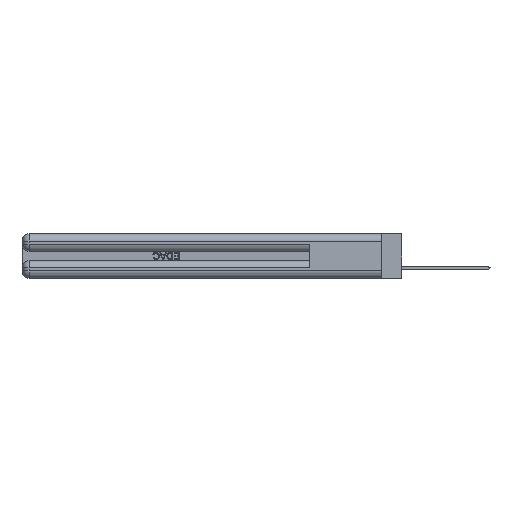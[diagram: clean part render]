
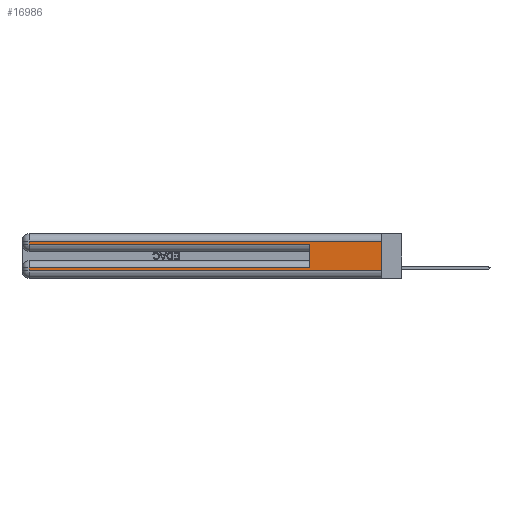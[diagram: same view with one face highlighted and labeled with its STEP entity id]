
A CAD part, left-side view. The second image highlights one B-rep face of the part: STEP entity #16986.
In plain terms, the highlighted planar face has unit normal (-1, 0, 0).
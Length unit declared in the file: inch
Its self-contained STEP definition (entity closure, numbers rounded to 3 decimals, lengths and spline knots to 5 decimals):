
#219 = EDGE_CURVE ( 'NONE', #20046, #39819, #32387, .T. ) ;
#1329 = ORIENTED_EDGE ( 'NONE', *, *, #219, .F. ) ;
#1887 = CARTESIAN_POINT ( 'NONE',  ( 0., 2.94, 0.37 ) ) ;
#1982 = AXIS2_PLACEMENT_3D ( 'NONE', #4326, #38796, #10562 ) ;
#2316 = CARTESIAN_POINT ( 'NONE',  ( 0., 0., 0.285 ) ) ;
#2643 = VECTOR ( 'NONE', #18544, 39.37008 ) ;
#3622 = DIRECTION ( 'NONE',  ( 0., 0., -1. ) ) ;
#4110 = VERTEX_POINT ( 'NONE', #21981 ) ;
#4326 = CARTESIAN_POINT ( 'NONE',  ( 0., 0., 0.37 ) ) ;
#4885 = VECTOR ( 'NONE', #17716, 39.37008 ) ;
#5286 = LINE ( 'NONE', #22515, #23518 ) ;
#6359 = ORIENTED_EDGE ( 'NONE', *, *, #16878, .T. ) ;
#6873 = VERTEX_POINT ( 'NONE', #15653 ) ;
#8966 = VERTEX_POINT ( 'NONE', #26097 ) ;
#9294 = ORIENTED_EDGE ( 'NONE', *, *, #29527, .T. ) ;
#9932 = EDGE_CURVE ( 'NONE', #8966, #39819, #20279, .T. ) ;
#10562 = DIRECTION ( 'NONE',  ( 0., 0., -1. ) ) ;
#11868 = VERTEX_POINT ( 'NONE', #23362 ) ;
#11932 = VECTOR ( 'NONE', #17241, 39.37008 ) ;
#13137 = ORIENTED_EDGE ( 'NONE', *, *, #9932, .T. ) ;
#13604 = DIRECTION ( 'NONE',  ( 0., 0., -1. ) ) ;
#14925 = VERTEX_POINT ( 'NONE', #15197 ) ;
#15197 = CARTESIAN_POINT ( 'NONE',  ( 0., 0.6, 0.285 ) ) ;
#15334 = VERTEX_POINT ( 'NONE', #21419 ) ;
#15653 = CARTESIAN_POINT ( 'NONE',  ( 0., 2.94, 0.085 ) ) ;
#16653 = PLANE ( 'NONE',  #1982 ) ;
#16878 = EDGE_CURVE ( 'NONE', #20046, #15334, #38776, .T. ) ;
#16986 = ADVANCED_FACE ( 'NONE', ( #18954 ), #16653, .F. ) ;
#17241 = DIRECTION ( 'NONE',  ( 0., -1., 0. ) ) ;
#17716 = DIRECTION ( 'NONE',  ( 0., -1., 0. ) ) ;
#18544 = DIRECTION ( 'NONE',  ( 0., 0., -1. ) ) ;
#18954 = FACE_OUTER_BOUND ( 'NONE', #26178, .T. ) ;
#20046 = VERTEX_POINT ( 'NONE', #40806 ) ;
#20279 = LINE ( 'NONE', #39378, #11932 ) ;
#20423 = LINE ( 'NONE', #1887, #2643 ) ;
#21126 = DIRECTION ( 'NONE',  ( 0., 0., 1. ) ) ;
#21419 = CARTESIAN_POINT ( 'NONE',  ( 0., 2.94, 0.31 ) ) ;
#21711 = LINE ( 'NONE', #2316, #4885 ) ;
#21981 = CARTESIAN_POINT ( 'NONE',  ( 0., 0.6, 0.085 ) ) ;
#22155 = EDGE_CURVE ( 'NONE', #15334, #11868, #20423, .T. ) ;
#22515 = CARTESIAN_POINT ( 'NONE',  ( 0., 0., 0.085 ) ) ;
#23362 = CARTESIAN_POINT ( 'NONE',  ( 0., 2.94, 0.285 ) ) ;
#23518 = VECTOR ( 'NONE', #38343, 39.37008 ) ;
#24508 = LINE ( 'NONE', #32663, #30419 ) ;
#24630 = CARTESIAN_POINT ( 'NONE',  ( 0., 0.6, 0.145 ) ) ;
#25377 = EDGE_CURVE ( 'NONE', #11868, #14925, #21711, .T. ) ;
#25508 = ORIENTED_EDGE ( 'NONE', *, *, #33144, .T. ) ;
#26097 = CARTESIAN_POINT ( 'NONE',  ( 0., 2.94, 0.06 ) ) ;
#26178 = EDGE_LOOP ( 'NONE', ( #1329, #6359, #27425, #26609, #29801, #9294, #25508, #13137 ) ) ;
#26609 = ORIENTED_EDGE ( 'NONE', *, *, #25377, .T. ) ;
#27210 = VECTOR ( 'NONE', #21126, 39.37008 ) ;
#27425 = ORIENTED_EDGE ( 'NONE', *, *, #22155, .T. ) ;
#27556 = EDGE_CURVE ( 'NONE', #4110, #14925, #35595, .T. ) ;
#29527 = EDGE_CURVE ( 'NONE', #4110, #6873, #5286, .T. ) ;
#29801 = ORIENTED_EDGE ( 'NONE', *, *, #27556, .F. ) ;
#30376 = VECTOR ( 'NONE', #34219, 39.37008 ) ;
#30419 = VECTOR ( 'NONE', #13604, 39.37008 ) ;
#30450 = CARTESIAN_POINT ( 'NONE',  ( 0., 0., 0.31 ) ) ;
#32270 = CARTESIAN_POINT ( 'NONE',  ( 0., 0., 0.37 ) ) ;
#32387 = LINE ( 'NONE', #32270, #36417 ) ;
#32663 = CARTESIAN_POINT ( 'NONE',  ( 0., 2.94, 0.37 ) ) ;
#33144 = EDGE_CURVE ( 'NONE', #6873, #8966, #24508, .T. ) ;
#34219 = DIRECTION ( 'NONE',  ( 0., 1., 0. ) ) ;
#34874 = CARTESIAN_POINT ( 'NONE',  ( 0., 0., 0.06 ) ) ;
#35595 = LINE ( 'NONE', #24630, #27210 ) ;
#36417 = VECTOR ( 'NONE', #3622, 39.37008 ) ;
#38343 = DIRECTION ( 'NONE',  ( 0., 1., 0. ) ) ;
#38776 = LINE ( 'NONE', #30450, #30376 ) ;
#38796 = DIRECTION ( 'NONE',  ( 1., 0., 0. ) ) ;
#39378 = CARTESIAN_POINT ( 'NONE',  ( 0., 0., 0.06 ) ) ;
#39819 = VERTEX_POINT ( 'NONE', #34874 ) ;
#40806 = CARTESIAN_POINT ( 'NONE',  ( 0., 0., 0.31 ) ) ;
